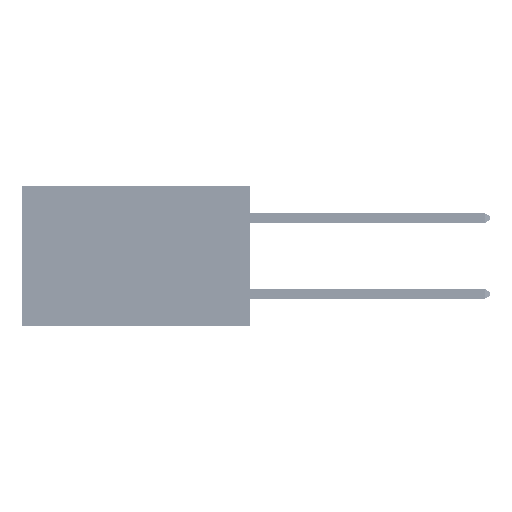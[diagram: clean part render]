
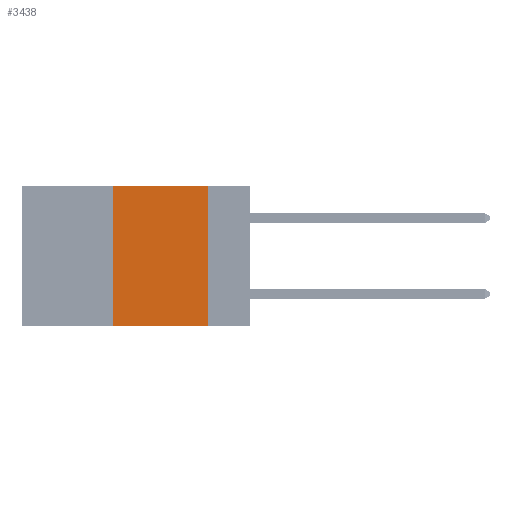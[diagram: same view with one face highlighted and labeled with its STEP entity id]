
A CAD part, left-side view. The second image highlights one B-rep face of the part: STEP entity #3438.
In plain terms, the highlighted planar face has unit normal (-1, 0, 0).
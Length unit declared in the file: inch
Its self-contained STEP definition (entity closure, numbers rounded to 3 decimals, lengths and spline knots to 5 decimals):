
#254 = VERTEX_POINT ( 'NONE', #38221 ) ;
#907 = CARTESIAN_POINT ( 'NONE',  ( 0., 0.11, 0. ) ) ;
#1798 = CARTESIAN_POINT ( 'NONE',  ( 0., 0.36, 0. ) ) ;
#2585 = ORIENTED_EDGE ( 'NONE', *, *, #52292, .F. ) ;
#2975 = ORIENTED_EDGE ( 'NONE', *, *, #35555, .T. ) ;
#3438 = ADVANCED_FACE ( 'NONE', ( #52553 ), #32474, .F. ) ;
#4605 = VECTOR ( 'NONE', #8367, 39.37008 ) ;
#6899 = CARTESIAN_POINT ( 'NONE',  ( 0., 0.36, -0.37 ) ) ;
#7572 = DIRECTION ( 'NONE',  ( 0., 0., -1. ) ) ;
#8367 = DIRECTION ( 'NONE',  ( 0., -1., 0. ) ) ;
#11743 = CARTESIAN_POINT ( 'NONE',  ( 0., 0.11, -0.37 ) ) ;
#11773 = EDGE_LOOP ( 'NONE', ( #40401, #2585, #16410, #2975 ) ) ;
#16410 = ORIENTED_EDGE ( 'NONE', *, *, #21097, .F. ) ;
#16896 = VERTEX_POINT ( 'NONE', #1798 ) ;
#19247 = DIRECTION ( 'NONE',  ( 0., 0., 1. ) ) ;
#21097 = EDGE_CURVE ( 'NONE', #31932, #16896, #46311, .T. ) ;
#23827 = VERTEX_POINT ( 'NONE', #11743 ) ;
#25788 = AXIS2_PLACEMENT_3D ( 'NONE', #46268, #53339, #7572 ) ;
#26145 = DIRECTION ( 'NONE',  ( 0., -1., 0. ) ) ;
#26377 = EDGE_CURVE ( 'NONE', #254, #23827, #33220, .T. ) ;
#26670 = CARTESIAN_POINT ( 'NONE',  ( 0., 0.6, 0. ) ) ;
#30045 = VECTOR ( 'NONE', #19247, 39.37008 ) ;
#31932 = VERTEX_POINT ( 'NONE', #6899 ) ;
#32474 = PLANE ( 'NONE',  #25788 ) ;
#33220 = LINE ( 'NONE', #907, #39054 ) ;
#33289 = CARTESIAN_POINT ( 'NONE',  ( 0., 0.6, -0.37 ) ) ;
#35049 = CARTESIAN_POINT ( 'NONE',  ( 0., 0.36, 0. ) ) ;
#35555 = EDGE_CURVE ( 'NONE', #31932, #23827, #39115, .T. ) ;
#36819 = VECTOR ( 'NONE', #26145, 39.37008 ) ;
#37469 = DIRECTION ( 'NONE',  ( 0., 0., -1. ) ) ;
#38221 = CARTESIAN_POINT ( 'NONE',  ( 0., 0.11, 0. ) ) ;
#39054 = VECTOR ( 'NONE', #37469, 39.37008 ) ;
#39115 = LINE ( 'NONE', #33289, #4605 ) ;
#40038 = LINE ( 'NONE', #26670, #36819 ) ;
#40401 = ORIENTED_EDGE ( 'NONE', *, *, #26377, .F. ) ;
#46268 = CARTESIAN_POINT ( 'NONE',  ( 0., 0.6, 0. ) ) ;
#46311 = LINE ( 'NONE', #35049, #30045 ) ;
#52292 = EDGE_CURVE ( 'NONE', #16896, #254, #40038, .T. ) ;
#52553 = FACE_OUTER_BOUND ( 'NONE', #11773, .T. ) ;
#53339 = DIRECTION ( 'NONE',  ( 1., 0., 0. ) ) ;
